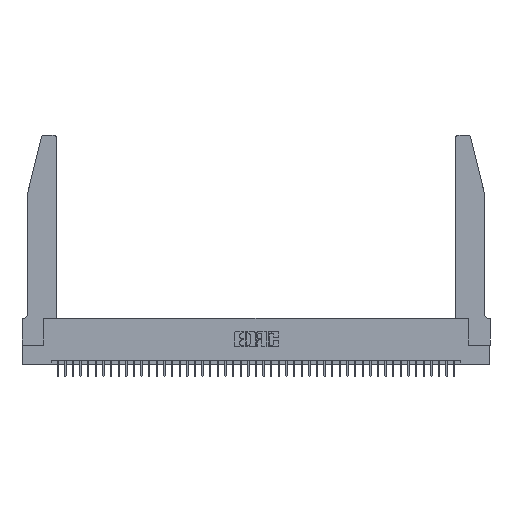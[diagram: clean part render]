
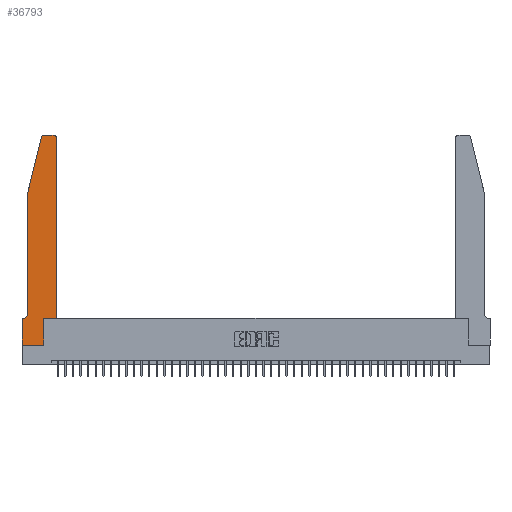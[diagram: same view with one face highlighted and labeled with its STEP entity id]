
A CAD part, top view. The second image highlights one B-rep face of the part: STEP entity #36793.
In plain terms, the highlighted planar face has unit normal (0, 0, 1).
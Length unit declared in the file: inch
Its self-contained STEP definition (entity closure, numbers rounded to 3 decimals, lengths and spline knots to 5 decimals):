
#242 = LINE ( 'NONE', #20929, #23637 ) ;
#442 = VERTEX_POINT ( 'NONE', #965 ) ;
#553 = DIRECTION ( 'NONE',  ( 0., -1., 0. ) ) ;
#770 = EDGE_CURVE ( 'NONE', #16803, #1361, #13687, .T. ) ;
#965 = CARTESIAN_POINT ( 'NONE',  ( 0.25487, 2.72718, 0.37 ) ) ;
#1139 = ORIENTED_EDGE ( 'NONE', *, *, #20335, .T. ) ;
#1361 = VERTEX_POINT ( 'NONE', #6995 ) ;
#1935 = CARTESIAN_POINT ( 'NONE',  ( 0.4505, 0.35, 0.37 ) ) ;
#1974 = CARTESIAN_POINT ( 'NONE',  ( 0.0055, 0.42, 0.37 ) ) ;
#2235 = EDGE_LOOP ( 'NONE', ( #21575, #24088, #4151, #8942, #25208, #14616, #24727, #6562, #1139, #12330, #41589, #3609 ) ) ;
#2266 = CARTESIAN_POINT ( 'NONE',  ( 0.0755, 2., 0.37 ) ) ;
#2293 = VECTOR ( 'NONE', #26064, 39.37008 ) ;
#2664 = DIRECTION ( 'NONE',  ( -1., 0., 0. ) ) ;
#3609 = ORIENTED_EDGE ( 'NONE', *, *, #27916, .T. ) ;
#3763 = EDGE_CURVE ( 'NONE', #9515, #7127, #38709, .T. ) ;
#4151 = ORIENTED_EDGE ( 'NONE', *, *, #33335, .T. ) ;
#4336 = AXIS2_PLACEMENT_3D ( 'NONE', #41817, #11846, #25203 ) ;
#5257 = LINE ( 'NONE', #12029, #21968 ) ;
#5557 = CARTESIAN_POINT ( 'NONE',  ( 0., 0.35, 0.37 ) ) ;
#6562 = ORIENTED_EDGE ( 'NONE', *, *, #30318, .T. ) ;
#6712 = EDGE_CURVE ( 'NONE', #17222, #9515, #10768, .T. ) ;
#6995 = CARTESIAN_POINT ( 'NONE',  ( 0., 0., 0.37 ) ) ;
#7127 = VERTEX_POINT ( 'NONE', #14668 ) ;
#8942 = ORIENTED_EDGE ( 'NONE', *, *, #6712, .T. ) ;
#9417 = VECTOR ( 'NONE', #20713, 39.37008 ) ;
#9515 = VERTEX_POINT ( 'NONE', #12913 ) ;
#10174 = EDGE_CURVE ( 'NONE', #29680, #31434, #24307, .T. ) ;
#10768 = LINE ( 'NONE', #2266, #2293 ) ;
#11207 = LINE ( 'NONE', #22119, #36805 ) ;
#11815 = DIRECTION ( 'NONE',  ( 1., 0., 0. ) ) ;
#11846 = DIRECTION ( 'NONE',  ( 0., 0., 1. ) ) ;
#11949 = CARTESIAN_POINT ( 'NONE',  ( 0.4505, 2.72, 0.37 ) ) ;
#12029 = CARTESIAN_POINT ( 'NONE',  ( 0.2865, 0.35, 0.37 ) ) ;
#12040 = CARTESIAN_POINT ( 'NONE',  ( 0.4205, 2.72, 0.37 ) ) ;
#12330 = ORIENTED_EDGE ( 'NONE', *, *, #38412, .T. ) ;
#12714 = DIRECTION ( 'NONE',  ( 0., 0., -1. ) ) ;
#12913 = CARTESIAN_POINT ( 'NONE',  ( 0.0755, 0.42, 0.37 ) ) ;
#13687 = LINE ( 'NONE', #17893, #33817 ) ;
#14001 = LINE ( 'NONE', #1935, #20523 ) ;
#14616 = ORIENTED_EDGE ( 'NONE', *, *, #39075, .T. ) ;
#14668 = CARTESIAN_POINT ( 'NONE',  ( 0.0055, 0.35, 0.37 ) ) ;
#14988 = VERTEX_POINT ( 'NONE', #31910 ) ;
#15351 = EDGE_CURVE ( 'NONE', #43263, #44804, #242, .T. ) ;
#16803 = VERTEX_POINT ( 'NONE', #5557 ) ;
#16893 = CARTESIAN_POINT ( 'NONE',  ( 0.0755, 2., 0.37 ) ) ;
#17222 = VERTEX_POINT ( 'NONE', #16893 ) ;
#17893 = CARTESIAN_POINT ( 'NONE',  ( 0., 0., 0.37 ) ) ;
#19783 = AXIS2_PLACEMENT_3D ( 'NONE', #44712, #23766, #44863 ) ;
#20335 = EDGE_CURVE ( 'NONE', #14988, #36505, #5257, .T. ) ;
#20494 = AXIS2_PLACEMENT_3D ( 'NONE', #1974, #12714, #39922 ) ;
#20523 = VECTOR ( 'NONE', #26207, 39.37008 ) ;
#20588 = EDGE_CURVE ( 'NONE', #31434, #442, #44855, .T. ) ;
#20713 = DIRECTION ( 'NONE',  ( -0.239, -0.971, 0. ) ) ;
#20929 = CARTESIAN_POINT ( 'NONE',  ( 0.4505, 0.35, 0.37 ) ) ;
#21024 = VECTOR ( 'NONE', #37353, 39.37008 ) ;
#21575 = ORIENTED_EDGE ( 'NONE', *, *, #10174, .T. ) ;
#21968 = VECTOR ( 'NONE', #36633, 39.37008 ) ;
#22119 = CARTESIAN_POINT ( 'NONE',  ( 0., 0., 0.37 ) ) ;
#22403 = LINE ( 'NONE', #41546, #9417 ) ;
#22520 = CARTESIAN_POINT ( 'NONE',  ( 0.284, 2.75, 0.37 ) ) ;
#23637 = VECTOR ( 'NONE', #35219, 39.37008 ) ;
#23766 = DIRECTION ( 'NONE',  ( 0., 0., 1. ) ) ;
#24088 = ORIENTED_EDGE ( 'NONE', *, *, #20588, .T. ) ;
#24307 = LINE ( 'NONE', #26484, #38984 ) ;
#24727 = ORIENTED_EDGE ( 'NONE', *, *, #770, .T. ) ;
#25203 = DIRECTION ( 'NONE',  ( 1., 0., 0. ) ) ;
#25208 = ORIENTED_EDGE ( 'NONE', *, *, #3763, .T. ) ;
#26064 = DIRECTION ( 'NONE',  ( 0., -1., 0. ) ) ;
#26092 = CARTESIAN_POINT ( 'NONE',  ( 0.0755, 0.35, 0.37 ) ) ;
#26207 = DIRECTION ( 'NONE',  ( 1., 0., 0. ) ) ;
#26484 = CARTESIAN_POINT ( 'NONE',  ( 0.2605, 2.75, 0.37 ) ) ;
#27846 = AXIS2_PLACEMENT_3D ( 'NONE', #12040, #36803, #36356 ) ;
#27916 = EDGE_CURVE ( 'NONE', #44804, #29680, #30235, .T. ) ;
#28917 = FACE_OUTER_BOUND ( 'NONE', #2235, .T. ) ;
#29680 = VERTEX_POINT ( 'NONE', #30265 ) ;
#30235 = CIRCLE ( 'NONE', #27846, 0.03 ) ;
#30265 = CARTESIAN_POINT ( 'NONE',  ( 0.4205, 2.75, 0.37 ) ) ;
#30318 = EDGE_CURVE ( 'NONE', #1361, #14988, #11207, .T. ) ;
#31434 = VERTEX_POINT ( 'NONE', #22520 ) ;
#31910 = CARTESIAN_POINT ( 'NONE',  ( 0.2865, 0., 0.37 ) ) ;
#33335 = EDGE_CURVE ( 'NONE', #442, #17222, #22403, .T. ) ;
#33817 = VECTOR ( 'NONE', #553, 39.37008 ) ;
#34217 = PLANE ( 'NONE',  #19783 ) ;
#35107 = LINE ( 'NONE', #26092, #21024 ) ;
#35219 = DIRECTION ( 'NONE',  ( 0., 1., 0. ) ) ;
#36356 = DIRECTION ( 'NONE',  ( 1., 0., 0. ) ) ;
#36505 = VERTEX_POINT ( 'NONE', #44307 ) ;
#36633 = DIRECTION ( 'NONE',  ( 0., 1., 0. ) ) ;
#36793 = ADVANCED_FACE ( 'NONE', ( #28917 ), #34217, .T. ) ;
#36803 = DIRECTION ( 'NONE',  ( 0., 0., 1. ) ) ;
#36805 = VECTOR ( 'NONE', #11815, 39.37008 ) ;
#37353 = DIRECTION ( 'NONE',  ( -1., 0., 0. ) ) ;
#38412 = EDGE_CURVE ( 'NONE', #36505, #43263, #14001, .T. ) ;
#38709 = CIRCLE ( 'NONE', #20494, 0.07 ) ;
#38984 = VECTOR ( 'NONE', #2664, 39.37008 ) ;
#39075 = EDGE_CURVE ( 'NONE', #7127, #16803, #35107, .T. ) ;
#39922 = DIRECTION ( 'NONE',  ( -1., 0., 0. ) ) ;
#41546 = CARTESIAN_POINT ( 'NONE',  ( 0.0755, 2., 0.37 ) ) ;
#41554 = CARTESIAN_POINT ( 'NONE',  ( 0.4505, 0.35, 0.37 ) ) ;
#41589 = ORIENTED_EDGE ( 'NONE', *, *, #15351, .T. ) ;
#41817 = CARTESIAN_POINT ( 'NONE',  ( 0.284, 2.72, 0.37 ) ) ;
#43263 = VERTEX_POINT ( 'NONE', #41554 ) ;
#44307 = CARTESIAN_POINT ( 'NONE',  ( 0.2865, 0.35, 0.37 ) ) ;
#44712 = CARTESIAN_POINT ( 'NONE',  ( 0., 0.35, 0.37 ) ) ;
#44804 = VERTEX_POINT ( 'NONE', #11949 ) ;
#44855 = CIRCLE ( 'NONE', #4336, 0.03 ) ;
#44863 = DIRECTION ( 'NONE',  ( 1., 0., 0. ) ) ;
